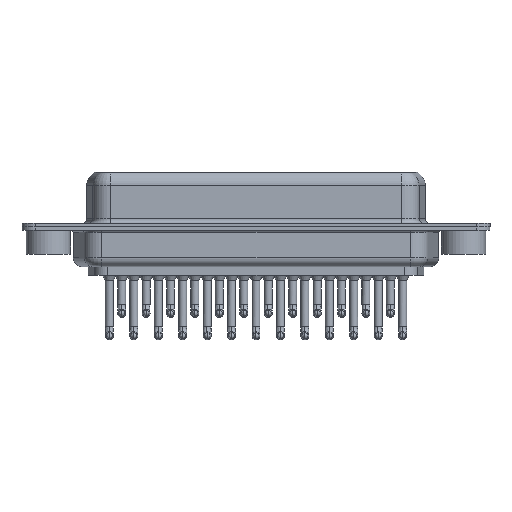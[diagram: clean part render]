
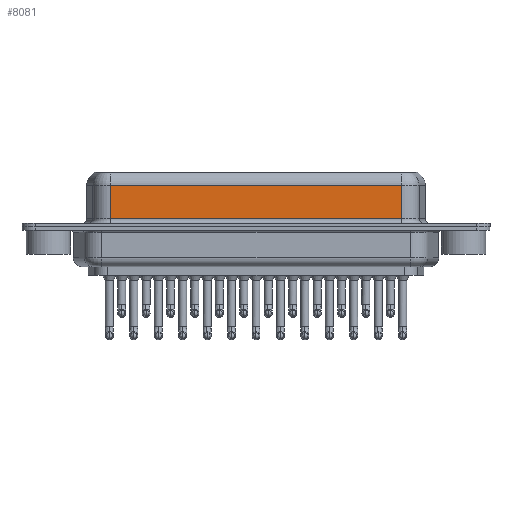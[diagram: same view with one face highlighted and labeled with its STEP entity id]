
A CAD part, front view. The second image highlights one B-rep face of the part: STEP entity #8081.
In plain terms, the highlighted planar face has unit normal (0, -1, 0).
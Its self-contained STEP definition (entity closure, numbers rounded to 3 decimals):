
#78 = CARTESIAN_POINT ( 'NONE',  ( 40.037, -3.95, 6.4 ) ) ;
#189 = ORIENTED_EDGE ( 'NONE', *, *, #1624, .T. ) ;
#774 = CARTESIAN_POINT ( 'NONE',  ( 40.037, -3.95, 0.9 ) ) ;
#1624 = EDGE_CURVE ( 'NONE', #17647, #21564, #8703, .T. ) ;
#1683 = EDGE_CURVE ( 'NONE', #17647, #20106, #21040, .T. ) ;
#1910 = FACE_OUTER_BOUND ( 'NONE', #19558, .T. ) ;
#2077 = VERTEX_POINT ( 'NONE', #12998 ) ;
#3397 = CARTESIAN_POINT ( 'NONE',  ( 40.037, -3.95, 0.9 ) ) ;
#5122 = DIRECTION ( 'NONE',  ( 1., 0., 0. ) ) ;
#5383 = CARTESIAN_POINT ( 'NONE',  ( 7.013, -3.95, 4.65 ) ) ;
#5425 = PLANE ( 'NONE',  #9046 ) ;
#7093 = DIRECTION ( 'NONE',  ( 0., 0., 1. ) ) ;
#8081 = ADVANCED_FACE ( 'NONE', ( #1910 ), #5425, .F. ) ;
#8703 = LINE ( 'NONE', #17891, #21602 ) ;
#9046 = AXIS2_PLACEMENT_3D ( 'NONE', #78, #16956, #7093 ) ;
#9473 = CARTESIAN_POINT ( 'NONE',  ( 7.013, -3.95, 6.4 ) ) ;
#11140 = DIRECTION ( 'NONE',  ( 0., 0., -1. ) ) ;
#12998 = CARTESIAN_POINT ( 'NONE',  ( 7.013, -3.95, 0.9 ) ) ;
#13124 = VECTOR ( 'NONE', #18665, 1000. ) ;
#14108 = ORIENTED_EDGE ( 'NONE', *, *, #20847, .T. ) ;
#14561 = CARTESIAN_POINT ( 'NONE',  ( 40.037, -3.95, 4.65 ) ) ;
#14725 = LINE ( 'NONE', #3397, #21672 ) ;
#16737 = VECTOR ( 'NONE', #11140, 1000. ) ;
#16956 = DIRECTION ( 'NONE',  ( 0., 1., 0. ) ) ;
#17647 = VERTEX_POINT ( 'NONE', #14561 ) ;
#17891 = CARTESIAN_POINT ( 'NONE',  ( 40.037, -3.95, 4.65 ) ) ;
#18110 = DIRECTION ( 'NONE',  ( -1., 0., 0. ) ) ;
#18651 = CARTESIAN_POINT ( 'NONE',  ( 40.037, -3.95, 6.4 ) ) ;
#18665 = DIRECTION ( 'NONE',  ( 0., 0., -1. ) ) ;
#18785 = ORIENTED_EDGE ( 'NONE', *, *, #20446, .T. ) ;
#19300 = ORIENTED_EDGE ( 'NONE', *, *, #1683, .F. ) ;
#19558 = EDGE_LOOP ( 'NONE', ( #19300, #189, #14108, #18785 ) ) ;
#20106 = VERTEX_POINT ( 'NONE', #774 ) ;
#20446 = EDGE_CURVE ( 'NONE', #2077, #20106, #14725, .T. ) ;
#20847 = EDGE_CURVE ( 'NONE', #21564, #2077, #21388, .T. ) ;
#21040 = LINE ( 'NONE', #18651, #13124 ) ;
#21388 = LINE ( 'NONE', #9473, #16737 ) ;
#21564 = VERTEX_POINT ( 'NONE', #5383 ) ;
#21602 = VECTOR ( 'NONE', #18110, 1000. ) ;
#21672 = VECTOR ( 'NONE', #5122, 1000. ) ;
